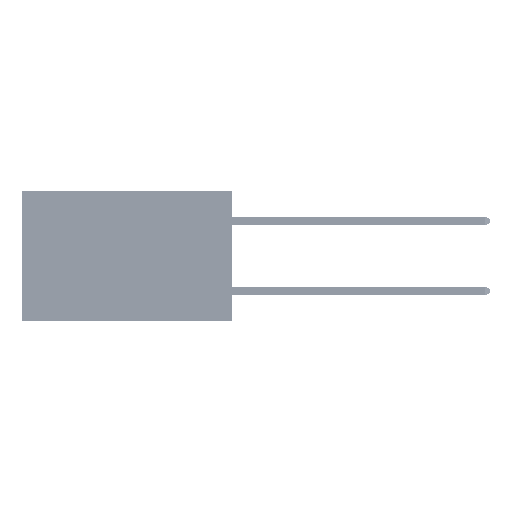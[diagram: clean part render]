
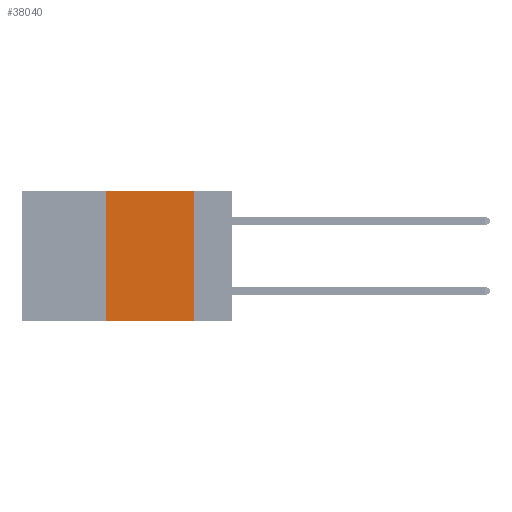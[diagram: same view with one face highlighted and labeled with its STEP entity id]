
A CAD part, left-side view. The second image highlights one B-rep face of the part: STEP entity #38040.
In plain terms, the highlighted planar face has unit normal (-1, 0, 0).
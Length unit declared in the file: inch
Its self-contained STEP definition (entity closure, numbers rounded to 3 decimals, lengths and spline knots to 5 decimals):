
#3115 = DIRECTION ( 'NONE',  ( 0., -1., 0. ) ) ;
#4765 = VERTEX_POINT ( 'NONE', #30213 ) ;
#7271 = EDGE_CURVE ( 'NONE', #32036, #4765, #16989, .T. ) ;
#7653 = PLANE ( 'NONE',  #38637 ) ;
#8175 = ORIENTED_EDGE ( 'NONE', *, *, #7271, .F. ) ;
#11048 = CARTESIAN_POINT ( 'NONE',  ( 0., 0.6, 0. ) ) ;
#12334 = VECTOR ( 'NONE', #47069, 39.37008 ) ;
#12354 = CARTESIAN_POINT ( 'NONE',  ( 0., 0.11, 0. ) ) ;
#13700 = VERTEX_POINT ( 'NONE', #18901 ) ;
#14351 = EDGE_LOOP ( 'NONE', ( #15000, #30823, #8175, #33276 ) ) ;
#15000 = ORIENTED_EDGE ( 'NONE', *, *, #47648, .F. ) ;
#16243 = DIRECTION ( 'NONE',  ( 1., 0., 0. ) ) ;
#16989 = LINE ( 'NONE', #49340, #43621 ) ;
#18901 = CARTESIAN_POINT ( 'NONE',  ( 0., 0.11, -0.37 ) ) ;
#22078 = CARTESIAN_POINT ( 'NONE',  ( 0., 0.36, -0.37 ) ) ;
#22177 = CARTESIAN_POINT ( 'NONE',  ( 0., 0.11, 0. ) ) ;
#23798 = LINE ( 'NONE', #11048, #12334 ) ;
#24762 = VERTEX_POINT ( 'NONE', #22177 ) ;
#27934 = CARTESIAN_POINT ( 'NONE',  ( 0., 0.6, 0. ) ) ;
#28217 = DIRECTION ( 'NONE',  ( 0., 0., -1. ) ) ;
#30213 = CARTESIAN_POINT ( 'NONE',  ( 0., 0.36, 0. ) ) ;
#30823 = ORIENTED_EDGE ( 'NONE', *, *, #42905, .F. ) ;
#31607 = FACE_OUTER_BOUND ( 'NONE', #14351, .T. ) ;
#32036 = VERTEX_POINT ( 'NONE', #22078 ) ;
#32872 = DIRECTION ( 'NONE',  ( 0., 0., 1. ) ) ;
#33276 = ORIENTED_EDGE ( 'NONE', *, *, #40966, .T. ) ;
#33332 = LINE ( 'NONE', #12354, #39194 ) ;
#35536 = VECTOR ( 'NONE', #3115, 39.37008 ) ;
#38040 = ADVANCED_FACE ( 'NONE', ( #31607 ), #7653, .F. ) ;
#38637 = AXIS2_PLACEMENT_3D ( 'NONE', #27934, #16243, #47821 ) ;
#39194 = VECTOR ( 'NONE', #28217, 39.37008 ) ;
#40966 = EDGE_CURVE ( 'NONE', #32036, #13700, #46958, .T. ) ;
#42905 = EDGE_CURVE ( 'NONE', #4765, #24762, #23798, .T. ) ;
#43621 = VECTOR ( 'NONE', #32872, 39.37008 ) ;
#46700 = CARTESIAN_POINT ( 'NONE',  ( 0., 0.6, -0.37 ) ) ;
#46958 = LINE ( 'NONE', #46700, #35536 ) ;
#47069 = DIRECTION ( 'NONE',  ( 0., -1., 0. ) ) ;
#47648 = EDGE_CURVE ( 'NONE', #24762, #13700, #33332, .T. ) ;
#47821 = DIRECTION ( 'NONE',  ( 0., 0., -1. ) ) ;
#49340 = CARTESIAN_POINT ( 'NONE',  ( 0., 0.36, 0. ) ) ;
